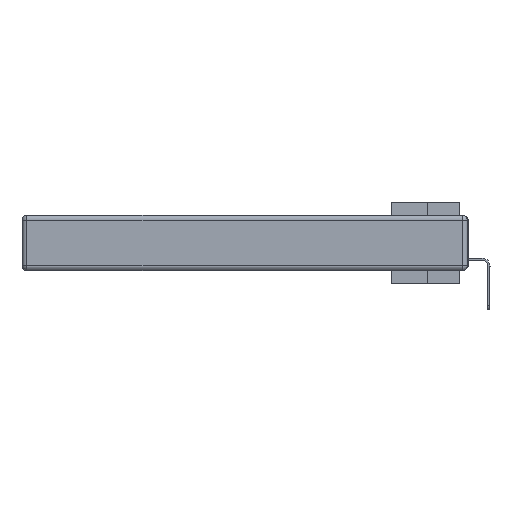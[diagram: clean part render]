
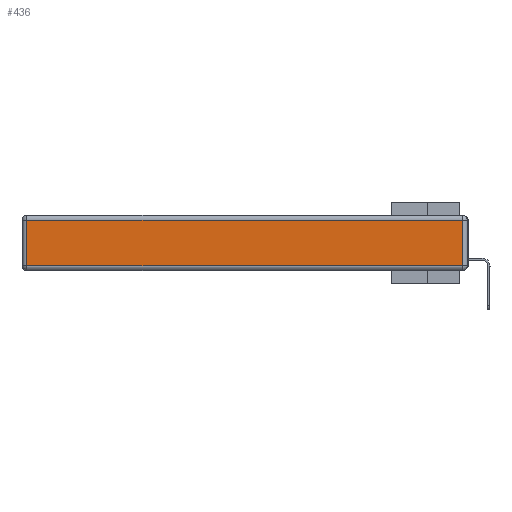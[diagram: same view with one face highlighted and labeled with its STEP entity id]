
A CAD part, left-side view. The second image highlights one B-rep face of the part: STEP entity #436.
In plain terms, the highlighted planar face has unit normal (-1, 0, 0).
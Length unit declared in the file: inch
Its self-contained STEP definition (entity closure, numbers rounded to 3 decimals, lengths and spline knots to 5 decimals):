
#1 = EDGE_CURVE ( 'NONE', #30293, #2531, #23884, .T. ) ;
#57 = VECTOR ( 'NONE', #17582, 39.37008 ) ;
#436 = ADVANCED_FACE ( 'NONE', ( #26014 ), #6263, .T. ) ;
#667 = ORIENTED_EDGE ( 'NONE', *, *, #24923, .T. ) ;
#897 = DIRECTION ( 'NONE',  ( -1., 0., 0. ) ) ;
#1242 = DIRECTION ( 'NONE',  ( 0., 1., 0. ) ) ;
#1885 = CARTESIAN_POINT ( 'NONE',  ( 0., 2.72, -0.03 ) ) ;
#1988 = CARTESIAN_POINT ( 'NONE',  ( 0., 0., -0.313 ) ) ;
#2531 = VERTEX_POINT ( 'NONE', #3284 ) ;
#3284 = CARTESIAN_POINT ( 'NONE',  ( 0., 0.03, -0.03 ) ) ;
#6263 = PLANE ( 'NONE',  #23089 ) ;
#6483 = CARTESIAN_POINT ( 'NONE',  ( 0., 0., -0.343 ) ) ;
#6728 = CARTESIAN_POINT ( 'NONE',  ( 0., 2.72, -0.313 ) ) ;
#9748 = VECTOR ( 'NONE', #25643, 39.37008 ) ;
#11631 = CARTESIAN_POINT ( 'NONE',  ( 0., 0.03, -0.313 ) ) ;
#11712 = CARTESIAN_POINT ( 'NONE',  ( 0., 2.75, -0.03 ) ) ;
#11924 = DIRECTION ( 'NONE',  ( 0., 0., -1. ) ) ;
#12874 = EDGE_LOOP ( 'NONE', ( #30491, #33433, #667, #30829 ) ) ;
#15325 = LINE ( 'NONE', #27860, #19504 ) ;
#16640 = EDGE_CURVE ( 'NONE', #17155, #30293, #20891, .T. ) ;
#17155 = VERTEX_POINT ( 'NONE', #6728 ) ;
#17582 = DIRECTION ( 'NONE',  ( 0., -1., 0. ) ) ;
#19504 = VECTOR ( 'NONE', #11924, 39.37008 ) ;
#20891 = LINE ( 'NONE', #1988, #57 ) ;
#22956 = CARTESIAN_POINT ( 'NONE',  ( 0., 0.03, -0.343 ) ) ;
#23089 = AXIS2_PLACEMENT_3D ( 'NONE', #6483, #897, #27532 ) ;
#23441 = VECTOR ( 'NONE', #1242, 39.37008 ) ;
#23884 = LINE ( 'NONE', #22956, #9748 ) ;
#24923 = EDGE_CURVE ( 'NONE', #2531, #28023, #27186, .T. ) ;
#25643 = DIRECTION ( 'NONE',  ( 0., 0., 1. ) ) ;
#26014 = FACE_OUTER_BOUND ( 'NONE', #12874, .T. ) ;
#27186 = LINE ( 'NONE', #11712, #23441 ) ;
#27532 = DIRECTION ( 'NONE',  ( 0., 0., 1. ) ) ;
#27860 = CARTESIAN_POINT ( 'NONE',  ( 0., 2.72, -0.343 ) ) ;
#28023 = VERTEX_POINT ( 'NONE', #1885 ) ;
#30293 = VERTEX_POINT ( 'NONE', #11631 ) ;
#30491 = ORIENTED_EDGE ( 'NONE', *, *, #16640, .T. ) ;
#30829 = ORIENTED_EDGE ( 'NONE', *, *, #33401, .T. ) ;
#33401 = EDGE_CURVE ( 'NONE', #28023, #17155, #15325, .T. ) ;
#33433 = ORIENTED_EDGE ( 'NONE', *, *, #1, .T. ) ;
